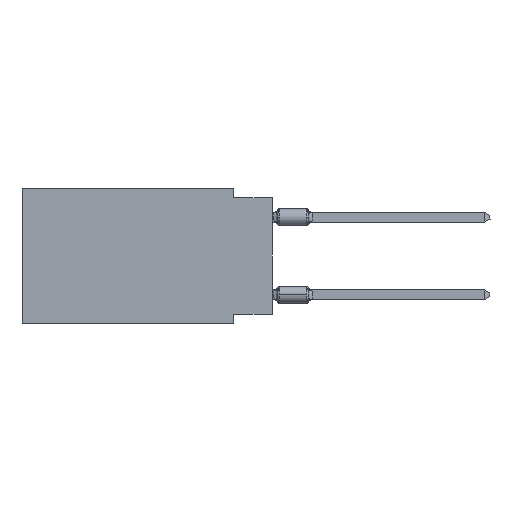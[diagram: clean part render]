
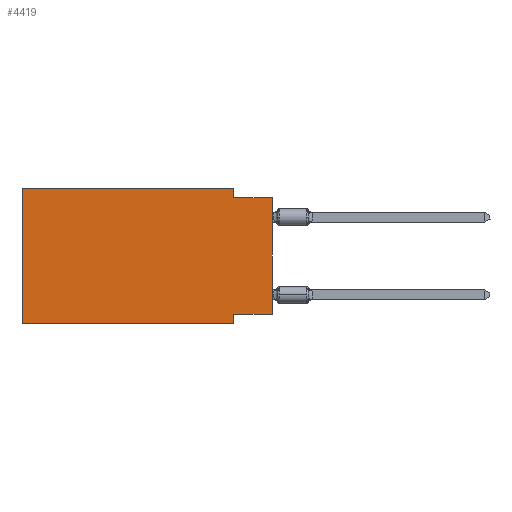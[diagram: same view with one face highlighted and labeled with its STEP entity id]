
A CAD part, left-side view. The second image highlights one B-rep face of the part: STEP entity #4419.
In plain terms, the highlighted planar face has unit normal (-1, 0, 0).
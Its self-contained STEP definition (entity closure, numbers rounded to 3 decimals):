
#740 = CARTESIAN_POINT ( 'NONE',  ( 0., 2.54, 0. ) ) ;
#806 = CARTESIAN_POINT ( 'NONE',  ( 0., 2.54, -8.255 ) ) ;
#1153 = DIRECTION ( 'NONE',  ( 0., -1., 0. ) ) ;
#1797 = VERTEX_POINT ( 'NONE', #27651 ) ;
#1893 = VERTEX_POINT ( 'NONE', #34973 ) ;
#1985 = FACE_OUTER_BOUND ( 'NONE', #29084, .T. ) ;
#2695 = CARTESIAN_POINT ( 'NONE',  ( 0., 0., -8.255 ) ) ;
#3423 = CARTESIAN_POINT ( 'NONE',  ( 0., 16.383, 0. ) ) ;
#4055 = CARTESIAN_POINT ( 'NONE',  ( 0., 0., -0.635 ) ) ;
#4419 = ADVANCED_FACE ( 'NONE', ( #1985 ), #31951, .F. ) ;
#4691 = CARTESIAN_POINT ( 'NONE',  ( 0., 16.383, 0. ) ) ;
#4885 = DIRECTION ( 'NONE',  ( 0., 0., -1. ) ) ;
#4945 = ORIENTED_EDGE ( 'NONE', *, *, #7355, .F. ) ;
#6268 = ORIENTED_EDGE ( 'NONE', *, *, #21579, .F. ) ;
#6297 = AXIS2_PLACEMENT_3D ( 'NONE', #4691, #31761, #4885 ) ;
#7355 = EDGE_CURVE ( 'NONE', #36915, #15590, #25981, .T. ) ;
#7507 = ORIENTED_EDGE ( 'NONE', *, *, #17028, .T. ) ;
#8323 = LINE ( 'NONE', #29381, #34382 ) ;
#8737 = DIRECTION ( 'NONE',  ( 0., 0., 1. ) ) ;
#8879 = CARTESIAN_POINT ( 'NONE',  ( 0., 2.54, -0.635 ) ) ;
#8927 = LINE ( 'NONE', #37563, #28920 ) ;
#9673 = LINE ( 'NONE', #4055, #10087 ) ;
#9863 = EDGE_CURVE ( 'NONE', #16617, #21557, #21447, .T. ) ;
#10087 = VECTOR ( 'NONE', #1153, 1000. ) ;
#10572 = CARTESIAN_POINT ( 'NONE',  ( 0., 16.383, -8.89 ) ) ;
#11482 = EDGE_CURVE ( 'NONE', #1797, #1893, #18689, .T. ) ;
#14571 = EDGE_CURVE ( 'NONE', #1797, #15590, #37061, .T. ) ;
#15204 = DIRECTION ( 'NONE',  ( 0., 0., 1. ) ) ;
#15590 = VERTEX_POINT ( 'NONE', #17923 ) ;
#16565 = DIRECTION ( 'NONE',  ( 0., -1., 0. ) ) ;
#16617 = VERTEX_POINT ( 'NONE', #20115 ) ;
#17028 = EDGE_CURVE ( 'NONE', #21499, #31010, #8927, .T. ) ;
#17923 = CARTESIAN_POINT ( 'NONE',  ( 0., 2.54, -8.89 ) ) ;
#18689 = LINE ( 'NONE', #3423, #19712 ) ;
#19503 = VECTOR ( 'NONE', #24116, 1000. ) ;
#19712 = VECTOR ( 'NONE', #15204, 1000. ) ;
#20115 = CARTESIAN_POINT ( 'NONE',  ( 0., 2.54, 0. ) ) ;
#20169 = VECTOR ( 'NONE', #38150, 1000. ) ;
#20867 = ORIENTED_EDGE ( 'NONE', *, *, #9863, .F. ) ;
#21223 = LINE ( 'NONE', #33010, #19503 ) ;
#21371 = VECTOR ( 'NONE', #16565, 1000. ) ;
#21424 = ORIENTED_EDGE ( 'NONE', *, *, #29062, .F. ) ;
#21447 = LINE ( 'NONE', #740, #33889 ) ;
#21499 = VERTEX_POINT ( 'NONE', #2695 ) ;
#21557 = VERTEX_POINT ( 'NONE', #8879 ) ;
#21579 = EDGE_CURVE ( 'NONE', #1893, #16617, #8323, .T. ) ;
#22313 = DIRECTION ( 'NONE',  ( 0., -1., 0. ) ) ;
#22902 = CARTESIAN_POINT ( 'NONE',  ( 0., 2.54, -8.89 ) ) ;
#24116 = DIRECTION ( 'NONE',  ( 0., 1., 0. ) ) ;
#25981 = LINE ( 'NONE', #22902, #20169 ) ;
#26418 = ORIENTED_EDGE ( 'NONE', *, *, #11482, .F. ) ;
#27245 = DIRECTION ( 'NONE',  ( 0., 0., -1. ) ) ;
#27651 = CARTESIAN_POINT ( 'NONE',  ( 0., 16.383, -8.89 ) ) ;
#28901 = CARTESIAN_POINT ( 'NONE',  ( 0., 0., -0.635 ) ) ;
#28920 = VECTOR ( 'NONE', #8737, 1000. ) ;
#29062 = EDGE_CURVE ( 'NONE', #21499, #36915, #21223, .T. ) ;
#29084 = EDGE_LOOP ( 'NONE', ( #7507, #36135, #20867, #6268, #26418, #29791, #4945, #21424 ) ) ;
#29381 = CARTESIAN_POINT ( 'NONE',  ( 0., 16.383, 0. ) ) ;
#29791 = ORIENTED_EDGE ( 'NONE', *, *, #14571, .T. ) ;
#31010 = VERTEX_POINT ( 'NONE', #28901 ) ;
#31761 = DIRECTION ( 'NONE',  ( 1., 0., 0. ) ) ;
#31951 = PLANE ( 'NONE',  #6297 ) ;
#33010 = CARTESIAN_POINT ( 'NONE',  ( 0., 0., -8.255 ) ) ;
#33889 = VECTOR ( 'NONE', #27245, 1000. ) ;
#34382 = VECTOR ( 'NONE', #22313, 1000. ) ;
#34973 = CARTESIAN_POINT ( 'NONE',  ( 0., 16.383, 0. ) ) ;
#36135 = ORIENTED_EDGE ( 'NONE', *, *, #37426, .F. ) ;
#36915 = VERTEX_POINT ( 'NONE', #806 ) ;
#37061 = LINE ( 'NONE', #10572, #21371 ) ;
#37426 = EDGE_CURVE ( 'NONE', #21557, #31010, #9673, .T. ) ;
#37563 = CARTESIAN_POINT ( 'NONE',  ( 0., 0., 0. ) ) ;
#38150 = DIRECTION ( 'NONE',  ( 0., 0., -1. ) ) ;
